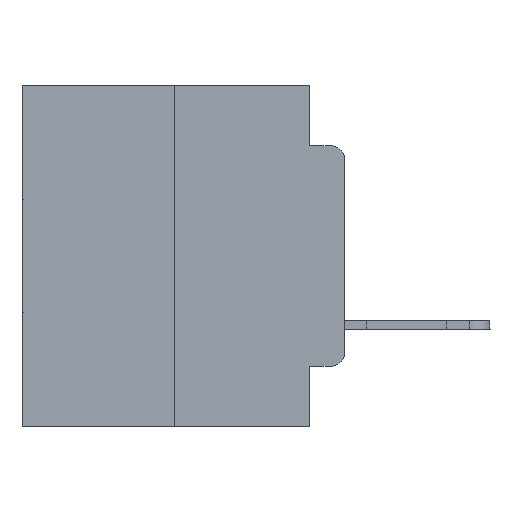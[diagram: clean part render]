
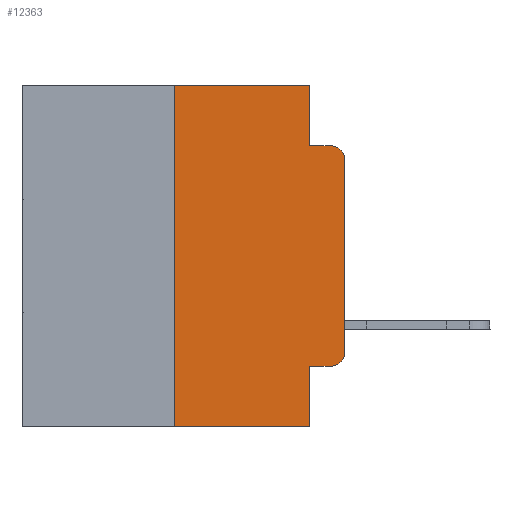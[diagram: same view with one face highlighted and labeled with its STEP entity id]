
A CAD part, left-side view. The second image highlights one B-rep face of the part: STEP entity #12363.
In plain terms, the highlighted planar face has unit normal (-1, 0, 0).
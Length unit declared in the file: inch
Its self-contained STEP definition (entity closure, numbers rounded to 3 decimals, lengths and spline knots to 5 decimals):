
#682 = CARTESIAN_POINT ( 'NONE',  ( 0., 0.051, 0. ) ) ;
#755 = DIRECTION ( 'NONE',  ( 0., -1., 0. ) ) ;
#1216 = CIRCLE ( 'NONE', #21153, 0.02 ) ;
#2116 = DIRECTION ( 'NONE',  ( 0., 0., 1. ) ) ;
#2801 = FACE_OUTER_BOUND ( 'NONE', #8825, .T. ) ;
#2919 = VERTEX_POINT ( 'NONE', #23144 ) ;
#3012 = DIRECTION ( 'NONE',  ( 0., 0., -1. ) ) ;
#3076 = PLANE ( 'NONE',  #10578 ) ;
#3117 = ORIENTED_EDGE ( 'NONE', *, *, #6542, .F. ) ;
#3409 = LINE ( 'NONE', #24657, #12626 ) ;
#3936 = ORIENTED_EDGE ( 'NONE', *, *, #12278, .T. ) ;
#4391 = CARTESIAN_POINT ( 'NONE',  ( 0., 0.473, -0.5 ) ) ;
#4404 = ORIENTED_EDGE ( 'NONE', *, *, #8144, .F. ) ;
#4613 = DIRECTION ( 'NONE',  ( -1., 0., 0. ) ) ;
#4777 = EDGE_CURVE ( 'NONE', #13031, #17875, #5428, .T. ) ;
#4994 = CARTESIAN_POINT ( 'NONE',  ( 0., 0.051, -0.5 ) ) ;
#5428 = LINE ( 'NONE', #9405, #22817 ) ;
#5698 = EDGE_CURVE ( 'NONE', #6334, #13682, #7338, .T. ) ;
#5735 = DIRECTION ( 'NONE',  ( 0., 0., -1. ) ) ;
#6334 = VERTEX_POINT ( 'NONE', #8288 ) ;
#6542 = EDGE_CURVE ( 'NONE', #7739, #27682, #6857, .T. ) ;
#6549 = ORIENTED_EDGE ( 'NONE', *, *, #5698, .F. ) ;
#6857 = LINE ( 'NONE', #15973, #14537 ) ;
#6938 = CARTESIAN_POINT ( 'NONE',  ( 0., 0.473, 0. ) ) ;
#7338 = LINE ( 'NONE', #682, #19908 ) ;
#7739 = VERTEX_POINT ( 'NONE', #24271 ) ;
#8144 = EDGE_CURVE ( 'NONE', #24864, #13031, #3409, .T. ) ;
#8288 = CARTESIAN_POINT ( 'NONE',  ( 0., 0.051, -0.4115 ) ) ;
#8505 = EDGE_CURVE ( 'NONE', #2919, #11787, #15483, .T. ) ;
#8667 = CARTESIAN_POINT ( 'NONE',  ( 0., 0., 0. ) ) ;
#8800 = DIRECTION ( 'NONE',  ( 0., -1., 0. ) ) ;
#8825 = EDGE_LOOP ( 'NONE', ( #22949, #17996, #3117, #14042, #14525, #4404, #3936, #6549, #25316, #19472 ) ) ;
#8948 = EDGE_CURVE ( 'NONE', #17875, #7739, #18360, .T. ) ;
#9405 = CARTESIAN_POINT ( 'NONE',  ( 0., 0.473, 0. ) ) ;
#9512 = VERTEX_POINT ( 'NONE', #25627 ) ;
#9726 = CARTESIAN_POINT ( 'NONE',  ( 0., 0.051, 0. ) ) ;
#9792 = DIRECTION ( 'NONE',  ( -1., 0., 0. ) ) ;
#9864 = EDGE_CURVE ( 'NONE', #11787, #27682, #1216, .T. ) ;
#10578 = AXIS2_PLACEMENT_3D ( 'NONE', #6938, #26451, #20386 ) ;
#10654 = LINE ( 'NONE', #4391, #12857 ) ;
#10868 = CARTESIAN_POINT ( 'NONE',  ( 0., 0.25, 0. ) ) ;
#11582 = CARTESIAN_POINT ( 'NONE',  ( 0., 0., -0.1085 ) ) ;
#11787 = VERTEX_POINT ( 'NONE', #11582 ) ;
#11821 = LINE ( 'NONE', #14229, #22436 ) ;
#12278 = EDGE_CURVE ( 'NONE', #24864, #13682, #10654, .T. ) ;
#12363 = ADVANCED_FACE ( 'NONE', ( #2801 ), #3076, .F. ) ;
#12626 = VECTOR ( 'NONE', #14226, 39.37008 ) ;
#12857 = VECTOR ( 'NONE', #8800, 39.37008 ) ;
#13031 = VERTEX_POINT ( 'NONE', #10868 ) ;
#13623 = CIRCLE ( 'NONE', #27118, 0.02 ) ;
#13682 = VERTEX_POINT ( 'NONE', #4994 ) ;
#14042 = ORIENTED_EDGE ( 'NONE', *, *, #8948, .F. ) ;
#14226 = DIRECTION ( 'NONE',  ( 0., 0., 1. ) ) ;
#14229 = CARTESIAN_POINT ( 'NONE',  ( 0., 0.051, -0.4115 ) ) ;
#14525 = ORIENTED_EDGE ( 'NONE', *, *, #4777, .F. ) ;
#14537 = VECTOR ( 'NONE', #755, 39.37008 ) ;
#15483 = LINE ( 'NONE', #8667, #16358 ) ;
#15919 = CARTESIAN_POINT ( 'NONE',  ( 0., 0.051, 0. ) ) ;
#15973 = CARTESIAN_POINT ( 'NONE',  ( 0., 0.051, -0.0885 ) ) ;
#16247 = EDGE_CURVE ( 'NONE', #6334, #9512, #11821, .T. ) ;
#16358 = VECTOR ( 'NONE', #2116, 39.37008 ) ;
#17875 = VERTEX_POINT ( 'NONE', #15919 ) ;
#17996 = ORIENTED_EDGE ( 'NONE', *, *, #9864, .T. ) ;
#18124 = DIRECTION ( 'NONE',  ( 0., 0., -1. ) ) ;
#18360 = LINE ( 'NONE', #9726, #21301 ) ;
#18382 = CARTESIAN_POINT ( 'NONE',  ( 0., 0.02, -0.0885 ) ) ;
#18426 = DIRECTION ( 'NONE',  ( 0., 0., -1. ) ) ;
#19472 = ORIENTED_EDGE ( 'NONE', *, *, #27895, .T. ) ;
#19908 = VECTOR ( 'NONE', #18124, 39.37008 ) ;
#20125 = CARTESIAN_POINT ( 'NONE',  ( 0., 0.02, -0.1085 ) ) ;
#20386 = DIRECTION ( 'NONE',  ( 0., 0., -1. ) ) ;
#20437 = DIRECTION ( 'NONE',  ( 0., -1., 0. ) ) ;
#21153 = AXIS2_PLACEMENT_3D ( 'NONE', #20125, #9792, #18426 ) ;
#21301 = VECTOR ( 'NONE', #5735, 39.37008 ) ;
#22436 = VECTOR ( 'NONE', #20437, 39.37008 ) ;
#22459 = CARTESIAN_POINT ( 'NONE',  ( 0., 0.02, -0.3915 ) ) ;
#22817 = VECTOR ( 'NONE', #24808, 39.37008 ) ;
#22949 = ORIENTED_EDGE ( 'NONE', *, *, #8505, .T. ) ;
#23144 = CARTESIAN_POINT ( 'NONE',  ( 0., 0., -0.3915 ) ) ;
#24271 = CARTESIAN_POINT ( 'NONE',  ( 0., 0.051, -0.0885 ) ) ;
#24657 = CARTESIAN_POINT ( 'NONE',  ( 0., 0.25, 0. ) ) ;
#24808 = DIRECTION ( 'NONE',  ( 0., -1., 0. ) ) ;
#24864 = VERTEX_POINT ( 'NONE', #26095 ) ;
#25316 = ORIENTED_EDGE ( 'NONE', *, *, #16247, .T. ) ;
#25627 = CARTESIAN_POINT ( 'NONE',  ( 0., 0.02, -0.4115 ) ) ;
#26095 = CARTESIAN_POINT ( 'NONE',  ( 0., 0.25, -0.5 ) ) ;
#26451 = DIRECTION ( 'NONE',  ( 1., 0., 0. ) ) ;
#27118 = AXIS2_PLACEMENT_3D ( 'NONE', #22459, #4613, #3012 ) ;
#27682 = VERTEX_POINT ( 'NONE', #18382 ) ;
#27895 = EDGE_CURVE ( 'NONE', #9512, #2919, #13623, .T. ) ;
